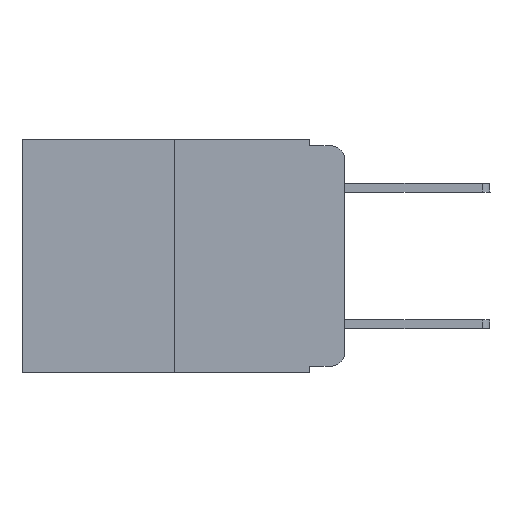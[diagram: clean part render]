
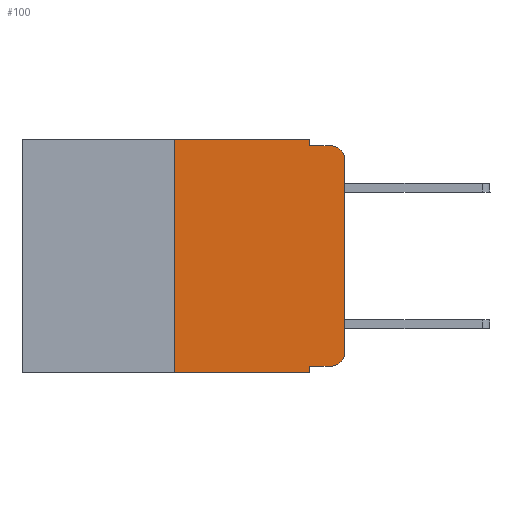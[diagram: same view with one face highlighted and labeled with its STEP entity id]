
A CAD part, left-side view. The second image highlights one B-rep face of the part: STEP entity #100.
In plain terms, the highlighted planar face has unit normal (-1, 0, 0).
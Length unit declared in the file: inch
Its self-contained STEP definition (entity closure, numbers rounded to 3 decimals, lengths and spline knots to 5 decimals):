
#92 = CARTESIAN_POINT ( 'NONE',  ( 0., 0.051, -0.333 ) ) ;
#100 = ADVANCED_FACE ( 'NONE', ( #18540 ), #16649, .F. ) ;
#264 = CARTESIAN_POINT ( 'NONE',  ( 0., 0.473, 0. ) ) ;
#416 = DIRECTION ( 'NONE',  ( 0., 0., 1. ) ) ;
#722 = CARTESIAN_POINT ( 'NONE',  ( 0., 0.051, -0.01 ) ) ;
#837 = CARTESIAN_POINT ( 'NONE',  ( 0., 0.02, -0.03 ) ) ;
#979 = EDGE_CURVE ( 'NONE', #12977, #18193, #4743, .T. ) ;
#1261 = DIRECTION ( 'NONE',  ( 0., 0., -1. ) ) ;
#1305 = DIRECTION ( 'NONE',  ( 0., -1., 0. ) ) ;
#1370 = CARTESIAN_POINT ( 'NONE',  ( 0., 0.473, 0. ) ) ;
#1382 = ORIENTED_EDGE ( 'NONE', *, *, #19478, .F. ) ;
#2563 = EDGE_CURVE ( 'NONE', #3247, #19615, #15702, .T. ) ;
#3247 = VERTEX_POINT ( 'NONE', #12865 ) ;
#3386 = EDGE_CURVE ( 'NONE', #20912, #3247, #13658, .T. ) ;
#3696 = CARTESIAN_POINT ( 'NONE',  ( 0., 0.25, 0. ) ) ;
#3735 = ORIENTED_EDGE ( 'NONE', *, *, #2563, .T. ) ;
#3918 = CARTESIAN_POINT ( 'NONE',  ( 0., 0.473, -0.343 ) ) ;
#3940 = EDGE_CURVE ( 'NONE', #12977, #20912, #13826, .T. ) ;
#4271 = VECTOR ( 'NONE', #5378, 39.37008 ) ;
#4311 = CARTESIAN_POINT ( 'NONE',  ( 0., 0.051, 0. ) ) ;
#4498 = VERTEX_POINT ( 'NONE', #7095 ) ;
#4669 = EDGE_CURVE ( 'NONE', #19615, #4498, #10761, .T. ) ;
#4743 = LINE ( 'NONE', #11546, #13262 ) ;
#4882 = VERTEX_POINT ( 'NONE', #18659 ) ;
#5378 = DIRECTION ( 'NONE',  ( 0., 0., 1. ) ) ;
#7095 = CARTESIAN_POINT ( 'NONE',  ( 0., 0.02, -0.01 ) ) ;
#7976 = VECTOR ( 'NONE', #10725, 39.37008 ) ;
#8330 = CARTESIAN_POINT ( 'NONE',  ( 0., 0.051, -0.01 ) ) ;
#8446 = LINE ( 'NONE', #8330, #16536 ) ;
#8702 = EDGE_CURVE ( 'NONE', #4882, #18193, #19188, .T. ) ;
#9420 = EDGE_CURVE ( 'NONE', #16515, #4498, #8446, .T. ) ;
#9634 = DIRECTION ( 'NONE',  ( -1., 0., 0. ) ) ;
#9737 = VECTOR ( 'NONE', #416, 39.37008 ) ;
#9965 = CARTESIAN_POINT ( 'NONE',  ( 0., 0.051, 0. ) ) ;
#10256 = ORIENTED_EDGE ( 'NONE', *, *, #4669, .T. ) ;
#10317 = LINE ( 'NONE', #264, #10980 ) ;
#10725 = DIRECTION ( 'NONE',  ( 0., -1., 0. ) ) ;
#10761 = CIRCLE ( 'NONE', #16446, 0.02 ) ;
#10980 = VECTOR ( 'NONE', #17100, 39.37008 ) ;
#11426 = DIRECTION ( 'NONE',  ( 0., 0., -1. ) ) ;
#11546 = CARTESIAN_POINT ( 'NONE',  ( 0., 0.051, 0. ) ) ;
#11805 = ORIENTED_EDGE ( 'NONE', *, *, #16080, .F. ) ;
#11882 = VERTEX_POINT ( 'NONE', #15939 ) ;
#12146 = AXIS2_PLACEMENT_3D ( 'NONE', #1370, #21423, #1261 ) ;
#12865 = CARTESIAN_POINT ( 'NONE',  ( 0., 0., -0.313 ) ) ;
#12977 = VERTEX_POINT ( 'NONE', #92 ) ;
#13189 = CARTESIAN_POINT ( 'NONE',  ( 0., 0.02, -0.313 ) ) ;
#13262 = VECTOR ( 'NONE', #18344, 39.37008 ) ;
#13406 = DIRECTION ( 'NONE',  ( 0., 0., -1. ) ) ;
#13658 = CIRCLE ( 'NONE', #16887, 0.02 ) ;
#13826 = LINE ( 'NONE', #16818, #21837 ) ;
#14083 = LINE ( 'NONE', #3696, #4271 ) ;
#14263 = VERTEX_POINT ( 'NONE', #9965 ) ;
#14426 = ORIENTED_EDGE ( 'NONE', *, *, #16381, .F. ) ;
#15325 = ORIENTED_EDGE ( 'NONE', *, *, #8702, .T. ) ;
#15672 = ORIENTED_EDGE ( 'NONE', *, *, #979, .F. ) ;
#15702 = LINE ( 'NONE', #19272, #9737 ) ;
#15939 = CARTESIAN_POINT ( 'NONE',  ( 0., 0.25, 0. ) ) ;
#15976 = ORIENTED_EDGE ( 'NONE', *, *, #9420, .F. ) ;
#16080 = EDGE_CURVE ( 'NONE', #14263, #16515, #19589, .T. ) ;
#16115 = ORIENTED_EDGE ( 'NONE', *, *, #3940, .T. ) ;
#16381 = EDGE_CURVE ( 'NONE', #11882, #14263, #10317, .T. ) ;
#16446 = AXIS2_PLACEMENT_3D ( 'NONE', #837, #19685, #11426 ) ;
#16515 = VERTEX_POINT ( 'NONE', #722 ) ;
#16536 = VECTOR ( 'NONE', #1305, 39.37008 ) ;
#16649 = PLANE ( 'NONE',  #12146 ) ;
#16818 = CARTESIAN_POINT ( 'NONE',  ( 0., 0.051, -0.333 ) ) ;
#16887 = AXIS2_PLACEMENT_3D ( 'NONE', #13189, #9634, #13406 ) ;
#16994 = CARTESIAN_POINT ( 'NONE',  ( 0., 0.02, -0.333 ) ) ;
#17100 = DIRECTION ( 'NONE',  ( 0., -1., 0. ) ) ;
#17544 = EDGE_LOOP ( 'NONE', ( #3735, #10256, #15976, #11805, #14426, #1382, #15325, #15672, #16115, #19095 ) ) ;
#18193 = VERTEX_POINT ( 'NONE', #21399 ) ;
#18344 = DIRECTION ( 'NONE',  ( 0., 0., -1. ) ) ;
#18448 = DIRECTION ( 'NONE',  ( 0., 0., -1. ) ) ;
#18540 = FACE_OUTER_BOUND ( 'NONE', #17544, .T. ) ;
#18659 = CARTESIAN_POINT ( 'NONE',  ( 0., 0.25, -0.343 ) ) ;
#18718 = DIRECTION ( 'NONE',  ( 0., -1., 0. ) ) ;
#18967 = CARTESIAN_POINT ( 'NONE',  ( 0., 0., -0.03 ) ) ;
#19095 = ORIENTED_EDGE ( 'NONE', *, *, #3386, .T. ) ;
#19188 = LINE ( 'NONE', #3918, #7976 ) ;
#19272 = CARTESIAN_POINT ( 'NONE',  ( 0., 0., 0. ) ) ;
#19478 = EDGE_CURVE ( 'NONE', #4882, #11882, #14083, .T. ) ;
#19589 = LINE ( 'NONE', #4311, #20538 ) ;
#19615 = VERTEX_POINT ( 'NONE', #18967 ) ;
#19685 = DIRECTION ( 'NONE',  ( -1., 0., 0. ) ) ;
#20538 = VECTOR ( 'NONE', #18448, 39.37008 ) ;
#20912 = VERTEX_POINT ( 'NONE', #16994 ) ;
#21399 = CARTESIAN_POINT ( 'NONE',  ( 0., 0.051, -0.343 ) ) ;
#21423 = DIRECTION ( 'NONE',  ( 1., 0., 0. ) ) ;
#21837 = VECTOR ( 'NONE', #18718, 39.37008 ) ;
